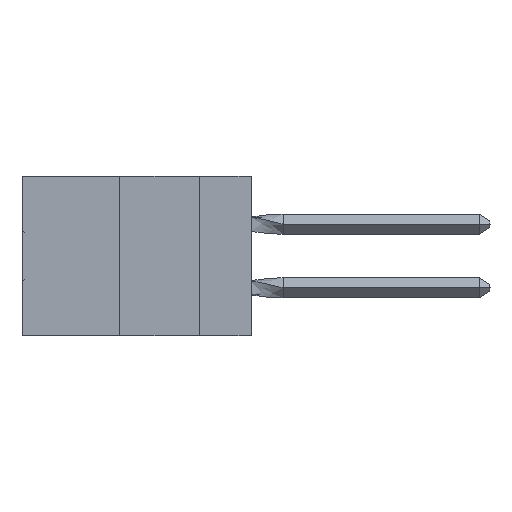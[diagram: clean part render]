
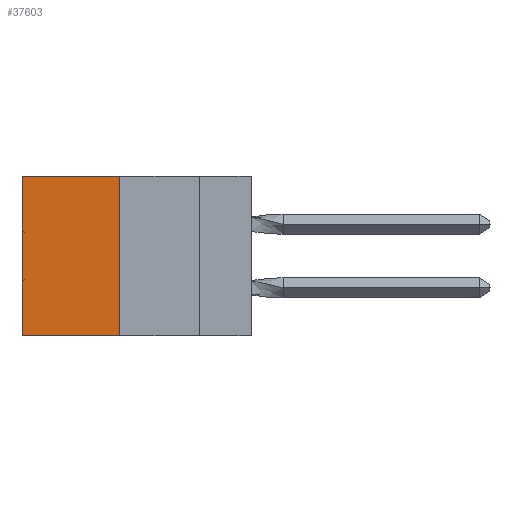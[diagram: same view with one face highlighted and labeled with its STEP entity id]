
A CAD part, left-side view. The second image highlights one B-rep face of the part: STEP entity #37603.
In plain terms, the highlighted planar face has unit normal (-1, 0, 0).
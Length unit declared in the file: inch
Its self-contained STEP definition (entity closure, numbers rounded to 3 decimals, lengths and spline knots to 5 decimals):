
#534 = ORIENTED_EDGE ( 'NONE', *, *, #27012, .T. ) ;
#1589 = VERTEX_POINT ( 'NONE', #24112 ) ;
#1878 = CARTESIAN_POINT ( 'NONE',  ( 0.305, 0.413, -0.5 ) ) ;
#4852 = CARTESIAN_POINT ( 'NONE',  ( 0.305, 0.413, -0.5 ) ) ;
#5389 = ORIENTED_EDGE ( 'NONE', *, *, #8686, .T. ) ;
#8444 = EDGE_CURVE ( 'NONE', #46080, #47326, #27223, .T. ) ;
#8686 = EDGE_CURVE ( 'NONE', #22762, #1589, #25375, .T. ) ;
#8892 = EDGE_LOOP ( 'NONE', ( #534, #45656, #33330, #5389 ) ) ;
#9778 = LINE ( 'NONE', #43663, #29226 ) ;
#12056 = DIRECTION ( 'NONE',  ( 0., 0., -1. ) ) ;
#14264 = DIRECTION ( 'NONE',  ( 0., 0., -1. ) ) ;
#16374 = FACE_OUTER_BOUND ( 'NONE', #8892, .T. ) ;
#17624 = CARTESIAN_POINT ( 'NONE',  ( 0.305, 0.72, -0.5 ) ) ;
#19745 = EDGE_CURVE ( 'NONE', #22762, #46080, #9778, .T. ) ;
#20355 = AXIS2_PLACEMENT_3D ( 'NONE', #4852, #23817, #12056 ) ;
#21050 = CARTESIAN_POINT ( 'NONE',  ( 0.305, 0.413, 0. ) ) ;
#22762 = VERTEX_POINT ( 'NONE', #21050 ) ;
#23817 = DIRECTION ( 'NONE',  ( 1., 0., 0. ) ) ;
#24112 = CARTESIAN_POINT ( 'NONE',  ( 0.305, 0.72, 0. ) ) ;
#25375 = LINE ( 'NONE', #29480, #27808 ) ;
#27012 = EDGE_CURVE ( 'NONE', #1589, #47326, #50317, .T. ) ;
#27223 = LINE ( 'NONE', #32236, #43759 ) ;
#27808 = VECTOR ( 'NONE', #49598, 39.37008 ) ;
#28033 = PLANE ( 'NONE',  #20355 ) ;
#29226 = VECTOR ( 'NONE', #43484, 39.37008 ) ;
#29480 = CARTESIAN_POINT ( 'NONE',  ( 0.305, 0.413, 0. ) ) ;
#29559 = VECTOR ( 'NONE', #14264, 39.37008 ) ;
#32236 = CARTESIAN_POINT ( 'NONE',  ( 0.305, 0.413, -0.5 ) ) ;
#33330 = ORIENTED_EDGE ( 'NONE', *, *, #19745, .F. ) ;
#37603 = ADVANCED_FACE ( 'NONE', ( #16374 ), #28033, .F. ) ;
#39807 = DIRECTION ( 'NONE',  ( 0., 1., 0. ) ) ;
#43484 = DIRECTION ( 'NONE',  ( 0., 0., -1. ) ) ;
#43663 = CARTESIAN_POINT ( 'NONE',  ( 0.305, 0.413, -0.5 ) ) ;
#43759 = VECTOR ( 'NONE', #39807, 39.37008 ) ;
#43960 = CARTESIAN_POINT ( 'NONE',  ( 0.305, 0.72, -0.5 ) ) ;
#45656 = ORIENTED_EDGE ( 'NONE', *, *, #8444, .F. ) ;
#46080 = VERTEX_POINT ( 'NONE', #1878 ) ;
#47326 = VERTEX_POINT ( 'NONE', #43960 ) ;
#49598 = DIRECTION ( 'NONE',  ( 0., 1., 0. ) ) ;
#50317 = LINE ( 'NONE', #17624, #29559 ) ;
